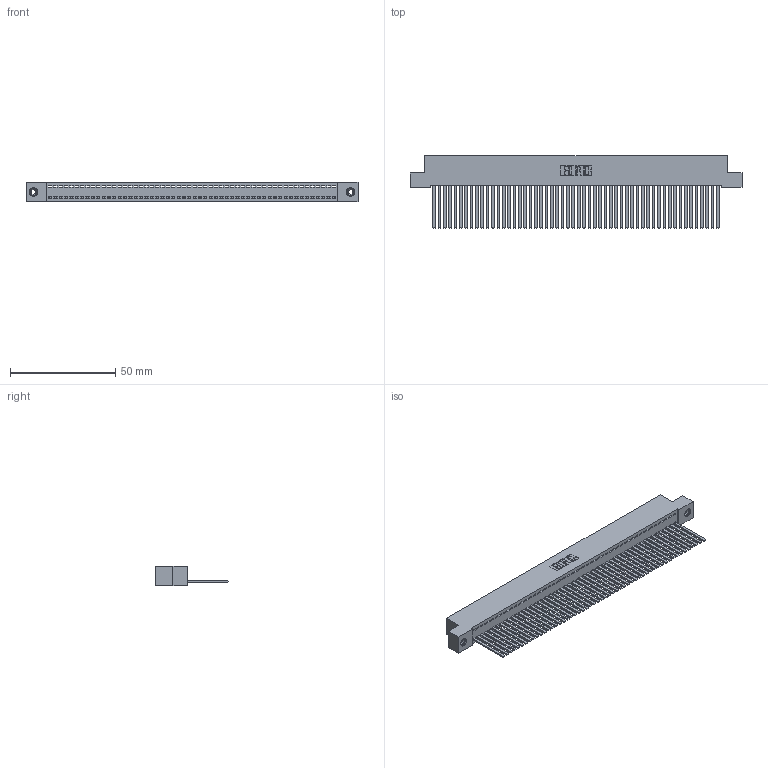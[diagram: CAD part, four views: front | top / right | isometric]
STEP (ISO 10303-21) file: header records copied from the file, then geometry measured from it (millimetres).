
FILE_DESCRIPTION (( 'STEP AP203' ), '1' );
FILE_NAME ('342-054-544-108.STEP', '2019-10-03T03:24:10', ( '' ), ( '' ), 'SwSTEP 2.0', 'SolidWorks 2016', '' );
FILE_SCHEMA (( 'CONFIG_CONTROL_DESIGN' ));
Length unit declared in the file: inch
Products named in the file (4): 342 Part_TI; 345-292-001_345-293-144; 345-250-001_345-250-003-102; 342-054-544-108
Assembly tree (57 placements, depth 2):
  342-054-544-108
    342 Part_TI
    345-292-001_345-293-144  x54
    345-250-001_345-250-003-102  x2
Bounding box: 157.48 x 34.3 x 9.4 mm (x, y, z)
Volume: 14471.8 mm3; surface area: 23272.9 mm2
Topology: 57 solids, 57 shells, 2978 faces, 8967 edges, 5898 vertices
Faces by surface type: plane 2150, cylinder 812, cone 12, torus 4
Entity records: 32330 total; most frequent: CARTESIAN_POINT 5555, ORIENTED_EDGE 5538, DIRECTION 4691, EDGE_CURVE 2769, LINE 2625, VECTOR 2625, VERTEX_POINT 1840, AXIS2_PLACEMENT_3D 1033
